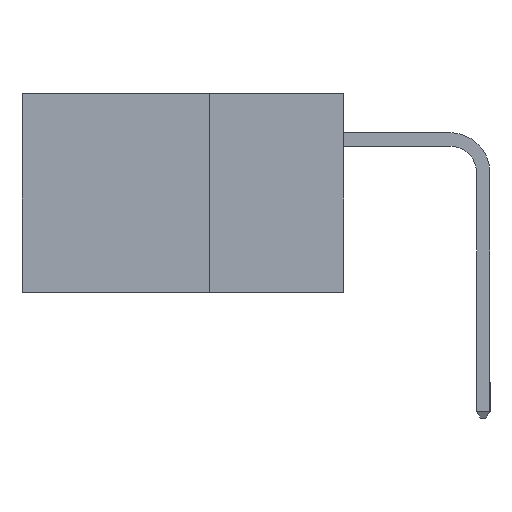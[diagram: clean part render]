
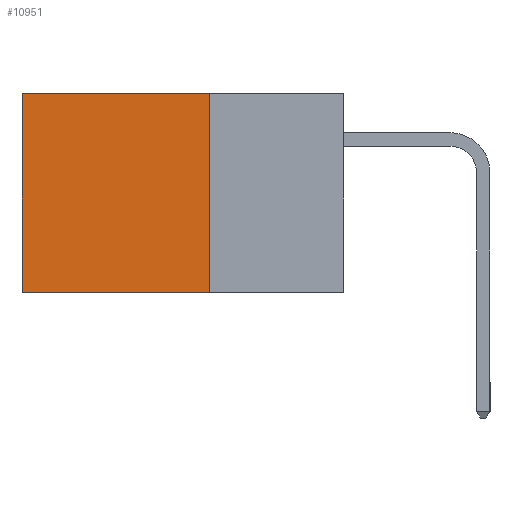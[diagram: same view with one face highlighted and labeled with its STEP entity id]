
A CAD part, left-side view. The second image highlights one B-rep face of the part: STEP entity #10951.
In plain terms, the highlighted planar face has unit normal (-1, 0, 0).
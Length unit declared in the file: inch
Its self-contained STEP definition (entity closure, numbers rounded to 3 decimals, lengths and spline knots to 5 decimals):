
#666 = CARTESIAN_POINT ( 'NONE',  ( 0.298, 0.25, 0. ) ) ;
#852 = VERTEX_POINT ( 'NONE', #666 ) ;
#1755 = AXIS2_PLACEMENT_3D ( 'NONE', #9925, #12955, #6944 ) ;
#1757 = CARTESIAN_POINT ( 'NONE',  ( 0.298, 0.25, 0. ) ) ;
#2264 = CARTESIAN_POINT ( 'NONE',  ( 0.298, 0.25, -0.37 ) ) ;
#3035 = DIRECTION ( 'NONE',  ( 0., 0., -1. ) ) ;
#3072 = FACE_OUTER_BOUND ( 'NONE', #5831, .T. ) ;
#3680 = EDGE_CURVE ( 'NONE', #852, #7366, #11352, .T. ) ;
#3778 = PLANE ( 'NONE',  #1755 ) ;
#4083 = LINE ( 'NONE', #10245, #11632 ) ;
#4880 = LINE ( 'NONE', #2264, #10040 ) ;
#5153 = VECTOR ( 'NONE', #9094, 39.37008 ) ;
#5752 = CARTESIAN_POINT ( 'NONE',  ( 0.298, 0.6, 0. ) ) ;
#5831 = EDGE_LOOP ( 'NONE', ( #10997, #12240, #12101, #10474 ) ) ;
#5927 = VECTOR ( 'NONE', #12050, 39.37008 ) ;
#6602 = CARTESIAN_POINT ( 'NONE',  ( 0.298, 0.6, -0.37 ) ) ;
#6944 = DIRECTION ( 'NONE',  ( 0., 0., -1. ) ) ;
#7366 = VERTEX_POINT ( 'NONE', #7726 ) ;
#7699 = CARTESIAN_POINT ( 'NONE',  ( 0.298, 0.25, 0. ) ) ;
#7726 = CARTESIAN_POINT ( 'NONE',  ( 0.298, 0.25, -0.37 ) ) ;
#7955 = LINE ( 'NONE', #1757, #5153 ) ;
#8098 = VERTEX_POINT ( 'NONE', #5752 ) ;
#9094 = DIRECTION ( 'NONE',  ( 0., 1., 0. ) ) ;
#9292 = VERTEX_POINT ( 'NONE', #6602 ) ;
#9596 = EDGE_CURVE ( 'NONE', #8098, #9292, #4083, .T. ) ;
#9925 = CARTESIAN_POINT ( 'NONE',  ( 0.298, 0.25, 0. ) ) ;
#10040 = VECTOR ( 'NONE', #10540, 39.37008 ) ;
#10140 = EDGE_CURVE ( 'NONE', #7366, #9292, #4880, .T. ) ;
#10245 = CARTESIAN_POINT ( 'NONE',  ( 0.298, 0.6, 0. ) ) ;
#10474 = ORIENTED_EDGE ( 'NONE', *, *, #12770, .T. ) ;
#10540 = DIRECTION ( 'NONE',  ( 0., 1., 0. ) ) ;
#10951 = ADVANCED_FACE ( 'NONE', ( #3072 ), #3778, .F. ) ;
#10997 = ORIENTED_EDGE ( 'NONE', *, *, #9596, .T. ) ;
#11352 = LINE ( 'NONE', #7699, #5927 ) ;
#11632 = VECTOR ( 'NONE', #3035, 39.37008 ) ;
#12050 = DIRECTION ( 'NONE',  ( 0., 0., -1. ) ) ;
#12101 = ORIENTED_EDGE ( 'NONE', *, *, #3680, .F. ) ;
#12240 = ORIENTED_EDGE ( 'NONE', *, *, #10140, .F. ) ;
#12770 = EDGE_CURVE ( 'NONE', #852, #8098, #7955, .T. ) ;
#12955 = DIRECTION ( 'NONE',  ( 1., 0., 0. ) ) ;
